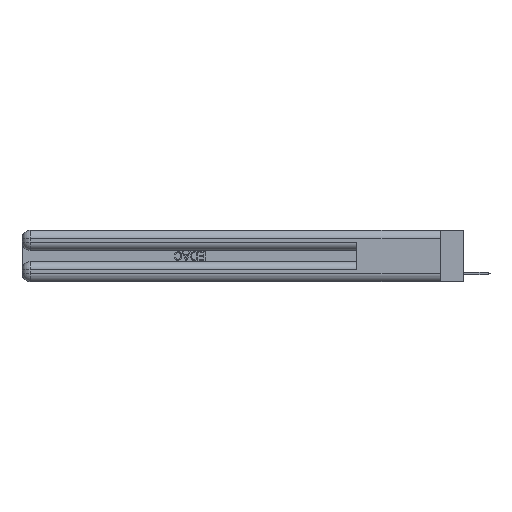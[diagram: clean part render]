
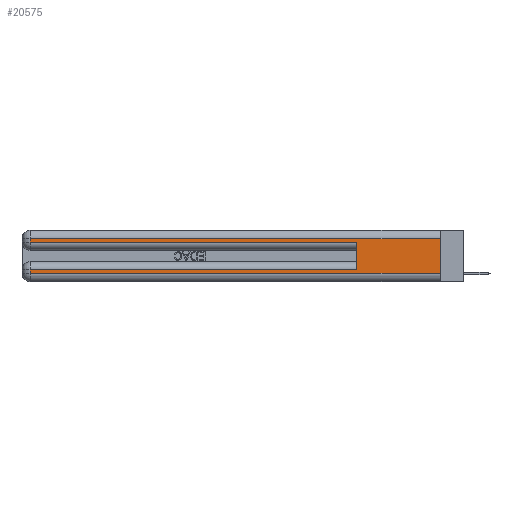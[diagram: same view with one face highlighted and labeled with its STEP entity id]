
A CAD part, left-side view. The second image highlights one B-rep face of the part: STEP entity #20575.
In plain terms, the highlighted planar face has unit normal (-1, 0, 0).
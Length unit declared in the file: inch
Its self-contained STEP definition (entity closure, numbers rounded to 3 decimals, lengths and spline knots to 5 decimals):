
#898 = CARTESIAN_POINT ( 'NONE',  ( 0., 2.94, 0.06 ) ) ;
#910 = LINE ( 'NONE', #27077, #24487 ) ;
#2172 = VERTEX_POINT ( 'NONE', #7772 ) ;
#2304 = CARTESIAN_POINT ( 'NONE',  ( 0., 0., 0.31 ) ) ;
#3093 = DIRECTION ( 'NONE',  ( 0., 0., -1. ) ) ;
#4107 = DIRECTION ( 'NONE',  ( 0., -1., 0. ) ) ;
#4155 = VERTEX_POINT ( 'NONE', #9366 ) ;
#4211 = CARTESIAN_POINT ( 'NONE',  ( 0., 0.6, 0.285 ) ) ;
#4602 = DIRECTION ( 'NONE',  ( 1., 0., 0. ) ) ;
#4679 = EDGE_CURVE ( 'NONE', #5447, #18145, #4862, .T. ) ;
#4862 = LINE ( 'NONE', #19660, #13128 ) ;
#4872 = DIRECTION ( 'NONE',  ( 0., 1., 0. ) ) ;
#4873 = DIRECTION ( 'NONE',  ( 0., 0., 1. ) ) ;
#5007 = DIRECTION ( 'NONE',  ( 0., -1., 0. ) ) ;
#5447 = VERTEX_POINT ( 'NONE', #8712 ) ;
#5621 = CARTESIAN_POINT ( 'NONE',  ( 0., 0., 0.285 ) ) ;
#5936 = LINE ( 'NONE', #5621, #9292 ) ;
#7019 = CARTESIAN_POINT ( 'NONE',  ( 0., 2.94, 0.37 ) ) ;
#7100 = ORIENTED_EDGE ( 'NONE', *, *, #15283, .F. ) ;
#7101 = VECTOR ( 'NONE', #4872, 39.37008 ) ;
#7174 = DIRECTION ( 'NONE',  ( 0., 0., -1. ) ) ;
#7772 = CARTESIAN_POINT ( 'NONE',  ( 0., 0., 0.06 ) ) ;
#8105 = EDGE_LOOP ( 'NONE', ( #7100, #16257, #30811, #15623, #22915, #16064, #21906, #8785 ) ) ;
#8712 = CARTESIAN_POINT ( 'NONE',  ( 0., 0.6, 0.085 ) ) ;
#8785 = ORIENTED_EDGE ( 'NONE', *, *, #29035, .T. ) ;
#9289 = EDGE_CURVE ( 'NONE', #15947, #30799, #19837, .T. ) ;
#9292 = VECTOR ( 'NONE', #5007, 39.37008 ) ;
#9294 = EDGE_CURVE ( 'NONE', #18145, #19577, #13449, .T. ) ;
#9366 = CARTESIAN_POINT ( 'NONE',  ( 0., 2.94, 0.285 ) ) ;
#9791 = DIRECTION ( 'NONE',  ( 0., 0., -1. ) ) ;
#9867 = EDGE_CURVE ( 'NONE', #30799, #4155, #11550, .T. ) ;
#11550 = LINE ( 'NONE', #11866, #18307 ) ;
#11866 = CARTESIAN_POINT ( 'NONE',  ( 0., 2.94, 0.37 ) ) ;
#13128 = VECTOR ( 'NONE', #26739, 39.37008 ) ;
#13449 = LINE ( 'NONE', #7019, #28801 ) ;
#14605 = CARTESIAN_POINT ( 'NONE',  ( 0., 0., 0.06 ) ) ;
#15113 = LINE ( 'NONE', #26654, #16248 ) ;
#15117 = CARTESIAN_POINT ( 'NONE',  ( 0., 2.94, 0.31 ) ) ;
#15283 = EDGE_CURVE ( 'NONE', #15947, #2172, #910, .T. ) ;
#15623 = ORIENTED_EDGE ( 'NONE', *, *, #21864, .T. ) ;
#15947 = VERTEX_POINT ( 'NONE', #20107 ) ;
#16064 = ORIENTED_EDGE ( 'NONE', *, *, #4679, .T. ) ;
#16248 = VECTOR ( 'NONE', #4873, 39.37008 ) ;
#16257 = ORIENTED_EDGE ( 'NONE', *, *, #9289, .T. ) ;
#18145 = VERTEX_POINT ( 'NONE', #22402 ) ;
#18200 = VECTOR ( 'NONE', #4107, 39.37008 ) ;
#18307 = VECTOR ( 'NONE', #9791, 39.37008 ) ;
#19058 = DIRECTION ( 'NONE',  ( 0., 0., -1. ) ) ;
#19107 = CARTESIAN_POINT ( 'NONE',  ( 0., 0., 0.37 ) ) ;
#19577 = VERTEX_POINT ( 'NONE', #898 ) ;
#19660 = CARTESIAN_POINT ( 'NONE',  ( 0., 0., 0.085 ) ) ;
#19837 = LINE ( 'NONE', #2304, #7101 ) ;
#20107 = CARTESIAN_POINT ( 'NONE',  ( 0., 0., 0.31 ) ) ;
#20575 = ADVANCED_FACE ( 'NONE', ( #21564 ), #21184, .F. ) ;
#21184 = PLANE ( 'NONE',  #27875 ) ;
#21564 = FACE_OUTER_BOUND ( 'NONE', #8105, .T. ) ;
#21864 = EDGE_CURVE ( 'NONE', #4155, #24063, #5936, .T. ) ;
#21906 = ORIENTED_EDGE ( 'NONE', *, *, #9294, .T. ) ;
#22402 = CARTESIAN_POINT ( 'NONE',  ( 0., 2.94, 0.085 ) ) ;
#22915 = ORIENTED_EDGE ( 'NONE', *, *, #30072, .F. ) ;
#24063 = VERTEX_POINT ( 'NONE', #4211 ) ;
#24487 = VECTOR ( 'NONE', #3093, 39.37008 ) ;
#25652 = LINE ( 'NONE', #14605, #18200 ) ;
#26654 = CARTESIAN_POINT ( 'NONE',  ( 0., 0.6, 0.145 ) ) ;
#26739 = DIRECTION ( 'NONE',  ( 0., 1., 0. ) ) ;
#27077 = CARTESIAN_POINT ( 'NONE',  ( 0., 0., 0.37 ) ) ;
#27875 = AXIS2_PLACEMENT_3D ( 'NONE', #19107, #4602, #7174 ) ;
#28801 = VECTOR ( 'NONE', #19058, 39.37008 ) ;
#29035 = EDGE_CURVE ( 'NONE', #19577, #2172, #25652, .T. ) ;
#30072 = EDGE_CURVE ( 'NONE', #5447, #24063, #15113, .T. ) ;
#30799 = VERTEX_POINT ( 'NONE', #15117 ) ;
#30811 = ORIENTED_EDGE ( 'NONE', *, *, #9867, .T. ) ;
